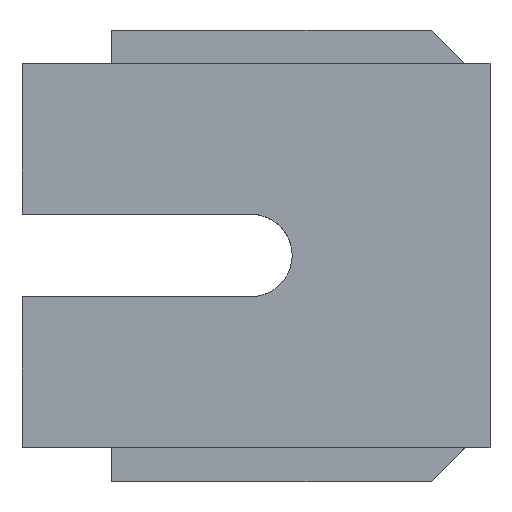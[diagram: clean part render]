
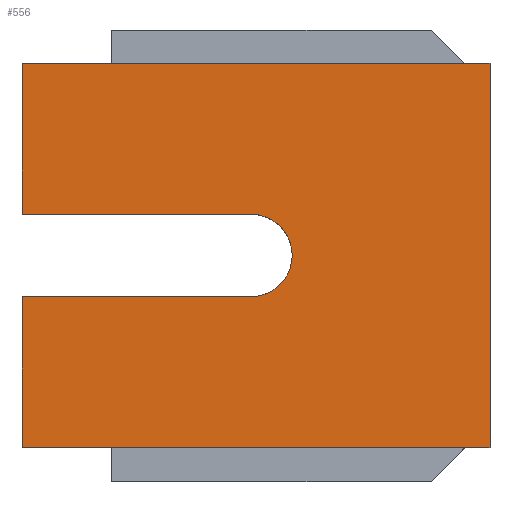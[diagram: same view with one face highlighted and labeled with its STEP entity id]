
A CAD part, top view. The second image highlights one B-rep face of the part: STEP entity #556.
In plain terms, the highlighted planar face has unit normal (0, 0, 1).
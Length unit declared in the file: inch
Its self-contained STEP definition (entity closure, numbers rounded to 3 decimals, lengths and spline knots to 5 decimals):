
#21=FACE_OUTER_BOUND('',#50,.T.);
#50=EDGE_LOOP('',(#368,#369,#370,#371,#372,#373,#374,#375));
#81=CIRCLE('',#606,0.08268);
#89=LINE('',#794,#161);
#90=LINE('',#796,#162);
#91=LINE('',#798,#163);
#92=LINE('',#800,#164);
#93=LINE('',#802,#165);
#94=LINE('',#804,#166);
#95=LINE('',#806,#167);
#161=VECTOR('',#646,0.3937);
#162=VECTOR('',#647,0.3937);
#163=VECTOR('',#648,0.3937);
#164=VECTOR('',#649,0.3937);
#165=VECTOR('',#650,0.3937);
#166=VECTOR('',#651,0.3937);
#167=VECTOR('',#652,0.3937);
#233=VERTEX_POINT('',#792);
#234=VERTEX_POINT('',#793);
#235=VERTEX_POINT('',#795);
#236=VERTEX_POINT('',#797);
#237=VERTEX_POINT('',#799);
#238=VERTEX_POINT('',#801);
#239=VERTEX_POINT('',#803);
#240=VERTEX_POINT('',#805);
#287=EDGE_CURVE('',#233,#234,#89,.T.);
#288=EDGE_CURVE('',#235,#234,#90,.T.);
#289=EDGE_CURVE('',#236,#235,#91,.T.);
#290=EDGE_CURVE('',#236,#237,#92,.T.);
#291=EDGE_CURVE('',#238,#237,#93,.T.);
#292=EDGE_CURVE('',#239,#238,#94,.T.);
#293=EDGE_CURVE('',#239,#240,#95,.T.);
#294=EDGE_CURVE('',#240,#233,#81,.T.);
#368=ORIENTED_EDGE('',*,*,#287,.T.);
#369=ORIENTED_EDGE('',*,*,#288,.F.);
#370=ORIENTED_EDGE('',*,*,#289,.F.);
#371=ORIENTED_EDGE('',*,*,#290,.T.);
#372=ORIENTED_EDGE('',*,*,#291,.F.);
#373=ORIENTED_EDGE('',*,*,#292,.F.);
#374=ORIENTED_EDGE('',*,*,#293,.T.);
#375=ORIENTED_EDGE('',*,*,#294,.T.);
#530=PLANE('',#605);
#556=ADVANCED_FACE('',(#21),#530,.T.);
#605=AXIS2_PLACEMENT_3D('',#791,#644,#645);
#606=AXIS2_PLACEMENT_3D('',#807,#653,#654);
#644=DIRECTION('center_axis',(0.,0.,1.));
#645=DIRECTION('ref_axis',(1.,0.,0.));
#646=DIRECTION('',(-1.,0.,0.));
#647=DIRECTION('',(0.,1.,0.));
#648=DIRECTION('',(-1.,0.,0.));
#649=DIRECTION('',(0.,1.,0.));
#650=DIRECTION('',(1.,0.,0.));
#651=DIRECTION('',(0.,1.,0.));
#652=DIRECTION('',(1.,0.,0.));
#653=DIRECTION('center_axis',(0.,0.,-1.));
#654=DIRECTION('ref_axis',(1.,0.,0.));
#791=CARTESIAN_POINT('Origin',(0.7874,0.,-1.02567));
#792=CARTESIAN_POINT('',(1.24701,-0.08268,-1.02567));
#793=CARTESIAN_POINT('',(0.7874,-0.08268,-1.02567));
#794=CARTESIAN_POINT('',(1.01228,-0.08268,-1.02567));
#795=CARTESIAN_POINT('',(0.7874,-0.38527,-1.02567));
#796=CARTESIAN_POINT('',(0.7874,0.,-1.02567));
#797=CARTESIAN_POINT('',(1.72657,-0.38527,-1.02567));
#798=CARTESIAN_POINT('',(1.72657,-0.38527,-1.02567));
#799=CARTESIAN_POINT('',(1.72657,0.38527,-1.02567));
#800=CARTESIAN_POINT('',(1.72657,0.,-1.02567));
#801=CARTESIAN_POINT('',(0.7874,0.38527,-1.02567));
#802=CARTESIAN_POINT('',(1.72657,0.38527,-1.02567));
#803=CARTESIAN_POINT('',(0.7874,0.08268,-1.02567));
#804=CARTESIAN_POINT('',(0.7874,0.,-1.02567));
#805=CARTESIAN_POINT('',(1.24701,0.08268,-1.02567));
#806=CARTESIAN_POINT('',(1.01228,0.08268,-1.02567));
#807=CARTESIAN_POINT('Origin',(1.24701,0.,-1.02567));
